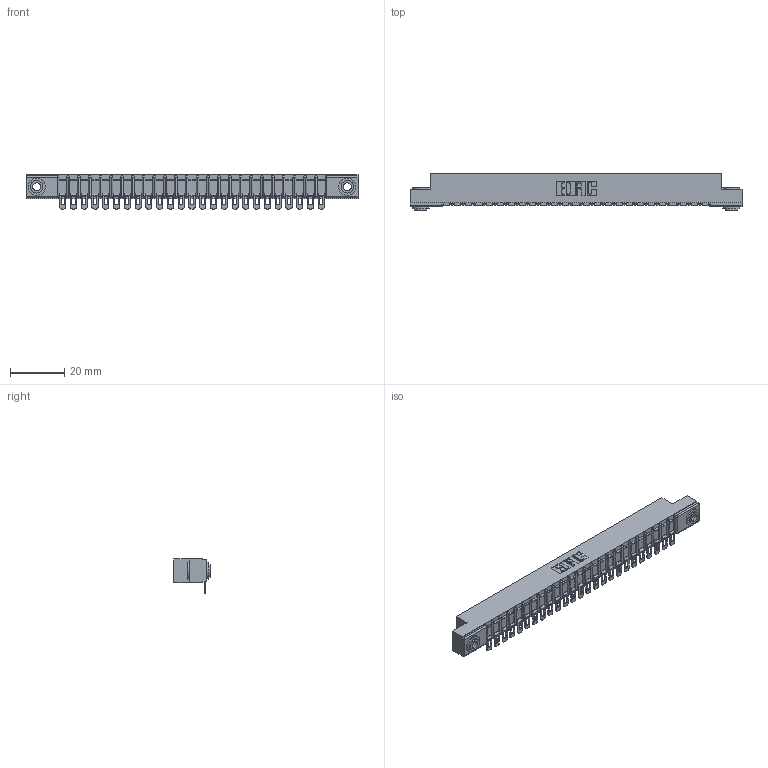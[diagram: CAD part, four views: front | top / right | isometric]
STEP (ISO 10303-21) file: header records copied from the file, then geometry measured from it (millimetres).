
FILE_DESCRIPTION (( 'STEP AP203' ), '1' );
FILE_NAME ('307-025-554-103.STEP', '2019-09-05T01:40:36', ( '' ), ( '' ), 'SwSTEP 2.0', 'SolidWorks 2016', '' );
FILE_SCHEMA (( 'CONFIG_CONTROL_DESIGN' ));
Length unit declared in the file: inch
Products named in the file (4): 307 Part_.156 Dia Mounting Holes; 345-250-002_345-250-002-102; 307-025-554-103; 307-290-002_554
Assembly tree (28 placements, depth 2):
  307-025-554-103
    307 Part_.156 Dia Mounting Holes
    307-290-002_554  x25
    345-250-002_345-250-002-102  x2
Bounding box: 122.07 x 13.36 x 12.52 mm (x, y, z)
Volume: 8070.9 mm3; surface area: 15193.2 mm2
Topology: 28 solids, 28 shells, 2221 faces, 6760 edges, 4432 vertices
Faces by surface type: plane 1244, cylinder 917, sphere 52, cone 8
Entity records: 25558 total; most frequent: CARTESIAN_POINT 4287, ORIENTED_EDGE 4268, DIRECTION 4194, EDGE_CURVE 2134, LINE 1612, VECTOR 1612, VERTEX_POINT 1384, AXIS2_PLACEMENT_3D 1291
